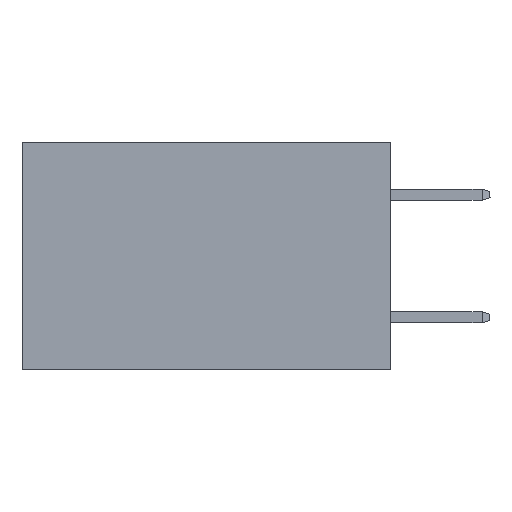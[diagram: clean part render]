
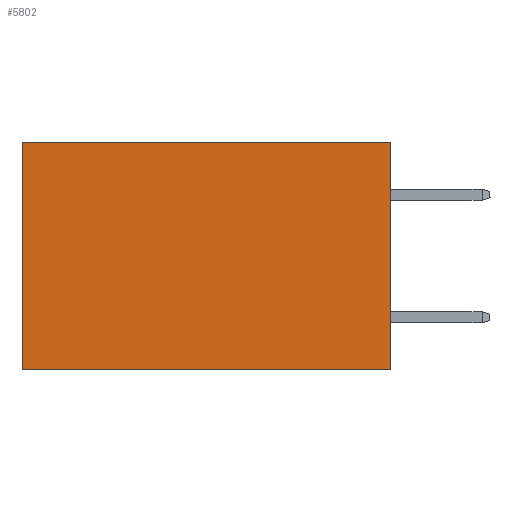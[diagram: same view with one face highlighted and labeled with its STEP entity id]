
A CAD part, left-side view. The second image highlights one B-rep face of the part: STEP entity #5802.
In plain terms, the highlighted planar face has unit normal (-1, 0, 0).
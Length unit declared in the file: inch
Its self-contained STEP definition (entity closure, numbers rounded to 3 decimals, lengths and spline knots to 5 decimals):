
#563 = VECTOR ( 'NONE', #5342, 39.37008 ) ;
#671 = CARTESIAN_POINT ( 'NONE',  ( 0.2875, 0., 0. ) ) ;
#810 = VERTEX_POINT ( 'NONE', #1709 ) ;
#1447 = ORIENTED_EDGE ( 'NONE', *, *, #3680, .F. ) ;
#1596 = ORIENTED_EDGE ( 'NONE', *, *, #3033, .T. ) ;
#1709 = CARTESIAN_POINT ( 'NONE',  ( 0.2875, 0., -0.37 ) ) ;
#1838 = ORIENTED_EDGE ( 'NONE', *, *, #14569, .T. ) ;
#2029 = EDGE_CURVE ( 'NONE', #810, #3570, #11528, .T. ) ;
#3033 = EDGE_CURVE ( 'NONE', #11310, #3570, #11810, .T. ) ;
#3570 = VERTEX_POINT ( 'NONE', #9256 ) ;
#3680 = EDGE_CURVE ( 'NONE', #6181, #810, #14757, .T. ) ;
#4156 = LINE ( 'NONE', #10896, #13147 ) ;
#4233 = CARTESIAN_POINT ( 'NONE',  ( 0.2875, 0.6, 0. ) ) ;
#4908 = CARTESIAN_POINT ( 'NONE',  ( 0.2875, 0., 0. ) ) ;
#5093 = ORIENTED_EDGE ( 'NONE', *, *, #2029, .F. ) ;
#5158 = FACE_OUTER_BOUND ( 'NONE', #7746, .T. ) ;
#5342 = DIRECTION ( 'NONE',  ( 0., 1., 0. ) ) ;
#5802 = ADVANCED_FACE ( 'NONE', ( #5158 ), #7280, .F. ) ;
#6039 = DIRECTION ( 'NONE',  ( 1., 0., 0. ) ) ;
#6181 = VERTEX_POINT ( 'NONE', #671 ) ;
#6626 = DIRECTION ( 'NONE',  ( 0., 0., -1. ) ) ;
#7280 = PLANE ( 'NONE',  #13880 ) ;
#7746 = EDGE_LOOP ( 'NONE', ( #1596, #5093, #1447, #1838 ) ) ;
#8433 = CARTESIAN_POINT ( 'NONE',  ( 0.2875, 0., 0. ) ) ;
#8864 = VECTOR ( 'NONE', #6626, 39.37008 ) ;
#9216 = CARTESIAN_POINT ( 'NONE',  ( 0.2875, 0.6, 0. ) ) ;
#9256 = CARTESIAN_POINT ( 'NONE',  ( 0.2875, 0.6, -0.37 ) ) ;
#9666 = DIRECTION ( 'NONE',  ( 0., 0., -1. ) ) ;
#10896 = CARTESIAN_POINT ( 'NONE',  ( 0.2875, 0., 0. ) ) ;
#11310 = VERTEX_POINT ( 'NONE', #4233 ) ;
#11528 = LINE ( 'NONE', #14771, #563 ) ;
#11810 = LINE ( 'NONE', #9216, #8864 ) ;
#12724 = VECTOR ( 'NONE', #14450, 39.37008 ) ;
#13147 = VECTOR ( 'NONE', #13311, 39.37008 ) ;
#13311 = DIRECTION ( 'NONE',  ( 0., 1., 0. ) ) ;
#13880 = AXIS2_PLACEMENT_3D ( 'NONE', #4908, #6039, #9666 ) ;
#14450 = DIRECTION ( 'NONE',  ( 0., 0., -1. ) ) ;
#14569 = EDGE_CURVE ( 'NONE', #6181, #11310, #4156, .T. ) ;
#14757 = LINE ( 'NONE', #8433, #12724 ) ;
#14771 = CARTESIAN_POINT ( 'NONE',  ( 0.2875, 0., -0.37 ) ) ;
